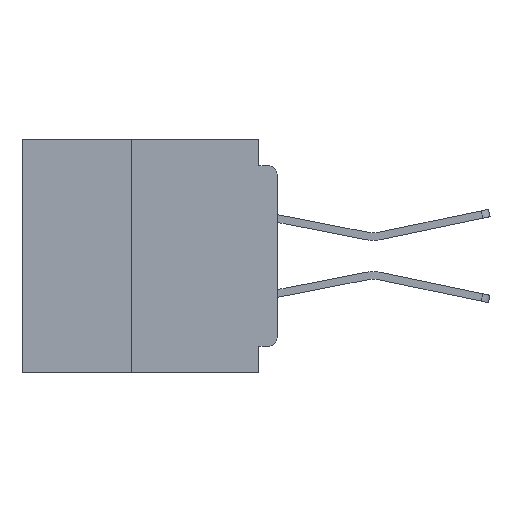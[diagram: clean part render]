
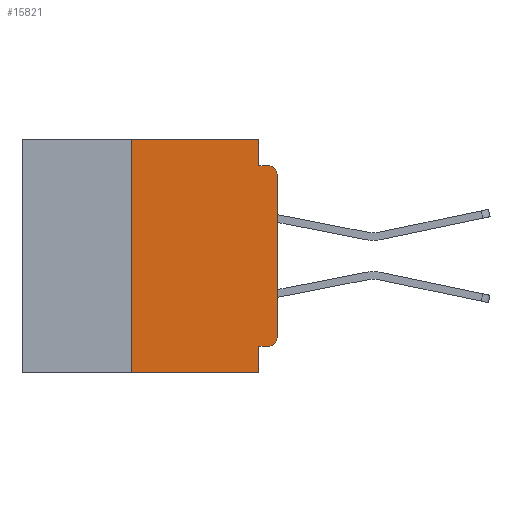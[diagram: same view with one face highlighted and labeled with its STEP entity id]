
A CAD part, left-side view. The second image highlights one B-rep face of the part: STEP entity #15821.
In plain terms, the highlighted planar face has unit normal (-1, 0, 0).
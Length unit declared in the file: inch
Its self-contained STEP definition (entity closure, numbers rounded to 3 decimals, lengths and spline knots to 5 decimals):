
#125 = CARTESIAN_POINT ( 'NONE',  ( 0., 0.437, 0. ) ) ;
#189 = LINE ( 'NONE', #2895, #1117 ) ;
#224 = ORIENTED_EDGE ( 'NONE', *, *, #13684, .T. ) ;
#247 = DIRECTION ( 'NONE',  ( 1., 0., 0. ) ) ;
#338 = DIRECTION ( 'NONE',  ( 0., -1., 0. ) ) ;
#1117 = VECTOR ( 'NONE', #5847, 39.37008 ) ;
#1561 = DIRECTION ( 'NONE',  ( -1., 0., 0. ) ) ;
#1771 = CARTESIAN_POINT ( 'NONE',  ( 0., 0.031, -0.4 ) ) ;
#2895 = CARTESIAN_POINT ( 'NONE',  ( 0., 0., 0. ) ) ;
#3011 = EDGE_CURVE ( 'NONE', #27664, #6868, #19219, .T. ) ;
#3291 = LINE ( 'NONE', #26087, #33215 ) ;
#4232 = CARTESIAN_POINT ( 'NONE',  ( 0., 0.25, 0. ) ) ;
#4723 = LINE ( 'NONE', #23804, #27044 ) ;
#4910 = EDGE_CURVE ( 'NONE', #15210, #10978, #12902, .T. ) ;
#5259 = LINE ( 'NONE', #9073, #35158 ) ;
#5656 = DIRECTION ( 'NONE',  ( 0., 0., -1. ) ) ;
#5847 = DIRECTION ( 'NONE',  ( 0., 0., 1. ) ) ;
#6216 = CARTESIAN_POINT ( 'NONE',  ( 0., 0.25, -0.4 ) ) ;
#6260 = CIRCLE ( 'NONE', #36345, 0.015 ) ;
#6534 = DIRECTION ( 'NONE',  ( 0., -1., 0. ) ) ;
#6868 = VERTEX_POINT ( 'NONE', #4232 ) ;
#7055 = VERTEX_POINT ( 'NONE', #35843 ) ;
#7603 = CARTESIAN_POINT ( 'NONE',  ( 0., 0.031, 0. ) ) ;
#7988 = ORIENTED_EDGE ( 'NONE', *, *, #3011, .F. ) ;
#8914 = VECTOR ( 'NONE', #30175, 39.37008 ) ;
#8932 = ORIENTED_EDGE ( 'NONE', *, *, #9797, .F. ) ;
#9073 = CARTESIAN_POINT ( 'NONE',  ( 0., 0.437, 0. ) ) ;
#9797 = EDGE_CURVE ( 'NONE', #30286, #15210, #9867, .T. ) ;
#9867 = LINE ( 'NONE', #21561, #8914 ) ;
#10670 = DIRECTION ( 'NONE',  ( 0., 0., 1. ) ) ;
#10978 = VERTEX_POINT ( 'NONE', #1771 ) ;
#11208 = ORIENTED_EDGE ( 'NONE', *, *, #34179, .F. ) ;
#11532 = VECTOR ( 'NONE', #10670, 39.37008 ) ;
#11995 = VECTOR ( 'NONE', #30623, 39.37008 ) ;
#12134 = ORIENTED_EDGE ( 'NONE', *, *, #4910, .F. ) ;
#12826 = DIRECTION ( 'NONE',  ( -1., 0., 0. ) ) ;
#12902 = LINE ( 'NONE', #31345, #11995 ) ;
#13684 = EDGE_CURVE ( 'NONE', #25320, #7055, #6260, .T. ) ;
#13890 = FACE_OUTER_BOUND ( 'NONE', #26585, .T. ) ;
#14215 = VERTEX_POINT ( 'NONE', #24144 ) ;
#14408 = DIRECTION ( 'NONE',  ( 0., -1., 0. ) ) ;
#14631 = LINE ( 'NONE', #31756, #15542 ) ;
#14784 = ORIENTED_EDGE ( 'NONE', *, *, #26121, .T. ) ;
#15210 = VERTEX_POINT ( 'NONE', #31455 ) ;
#15542 = VECTOR ( 'NONE', #14408, 39.37008 ) ;
#15813 = AXIS2_PLACEMENT_3D ( 'NONE', #30221, #12826, #33575 ) ;
#15821 = ADVANCED_FACE ( 'NONE', ( #13890 ), #34906, .F. ) ;
#17601 = AXIS2_PLACEMENT_3D ( 'NONE', #125, #247, #20554 ) ;
#18916 = CARTESIAN_POINT ( 'NONE',  ( 0., 0.015, -0.06 ) ) ;
#19219 = LINE ( 'NONE', #6216, #11532 ) ;
#19475 = CIRCLE ( 'NONE', #15813, 0.015 ) ;
#20554 = DIRECTION ( 'NONE',  ( 0., 0., -1. ) ) ;
#21561 = CARTESIAN_POINT ( 'NONE',  ( 0., 0., -0.355 ) ) ;
#21890 = DIRECTION ( 'NONE',  ( 0., 0., -1. ) ) ;
#23432 = EDGE_CURVE ( 'NONE', #30286, #14215, #19475, .T. ) ;
#23804 = CARTESIAN_POINT ( 'NONE',  ( 0., 0., -0.045 ) ) ;
#23981 = ORIENTED_EDGE ( 'NONE', *, *, #36635, .T. ) ;
#24144 = CARTESIAN_POINT ( 'NONE',  ( 0., 0., -0.34 ) ) ;
#24457 = VERTEX_POINT ( 'NONE', #35712 ) ;
#24943 = ORIENTED_EDGE ( 'NONE', *, *, #23432, .T. ) ;
#25026 = CARTESIAN_POINT ( 'NONE',  ( 0., 0.25, -0.4 ) ) ;
#25307 = ORIENTED_EDGE ( 'NONE', *, *, #35666, .F. ) ;
#25320 = VERTEX_POINT ( 'NONE', #25468 ) ;
#25468 = CARTESIAN_POINT ( 'NONE',  ( 0., 0., -0.06 ) ) ;
#25918 = CARTESIAN_POINT ( 'NONE',  ( 0., 0.015, -0.355 ) ) ;
#26087 = CARTESIAN_POINT ( 'NONE',  ( 0., 0.031, 0. ) ) ;
#26121 = EDGE_CURVE ( 'NONE', #14215, #25320, #189, .T. ) ;
#26585 = EDGE_LOOP ( 'NONE', ( #14784, #224, #25307, #29793, #11208, #7988, #23981, #12134, #8932, #24943 ) ) ;
#26931 = VERTEX_POINT ( 'NONE', #7603 ) ;
#27044 = VECTOR ( 'NONE', #6534, 39.37008 ) ;
#27128 = EDGE_CURVE ( 'NONE', #26931, #24457, #3291, .T. ) ;
#27664 = VERTEX_POINT ( 'NONE', #25026 ) ;
#29793 = ORIENTED_EDGE ( 'NONE', *, *, #27128, .F. ) ;
#30175 = DIRECTION ( 'NONE',  ( 0., 1., 0. ) ) ;
#30221 = CARTESIAN_POINT ( 'NONE',  ( 0., 0.015, -0.34 ) ) ;
#30286 = VERTEX_POINT ( 'NONE', #25918 ) ;
#30623 = DIRECTION ( 'NONE',  ( 0., 0., -1. ) ) ;
#31345 = CARTESIAN_POINT ( 'NONE',  ( 0., 0.031, -0.4 ) ) ;
#31455 = CARTESIAN_POINT ( 'NONE',  ( 0., 0.031, -0.355 ) ) ;
#31756 = CARTESIAN_POINT ( 'NONE',  ( 0., 0.437, -0.4 ) ) ;
#33215 = VECTOR ( 'NONE', #5656, 39.37008 ) ;
#33575 = DIRECTION ( 'NONE',  ( 0., 0., -1. ) ) ;
#34179 = EDGE_CURVE ( 'NONE', #6868, #26931, #5259, .T. ) ;
#34906 = PLANE ( 'NONE',  #17601 ) ;
#35158 = VECTOR ( 'NONE', #338, 39.37008 ) ;
#35666 = EDGE_CURVE ( 'NONE', #24457, #7055, #4723, .T. ) ;
#35712 = CARTESIAN_POINT ( 'NONE',  ( 0., 0.031, -0.045 ) ) ;
#35843 = CARTESIAN_POINT ( 'NONE',  ( 0., 0.015, -0.045 ) ) ;
#36345 = AXIS2_PLACEMENT_3D ( 'NONE', #18916, #1561, #21890 ) ;
#36635 = EDGE_CURVE ( 'NONE', #27664, #10978, #14631, .T. ) ;
